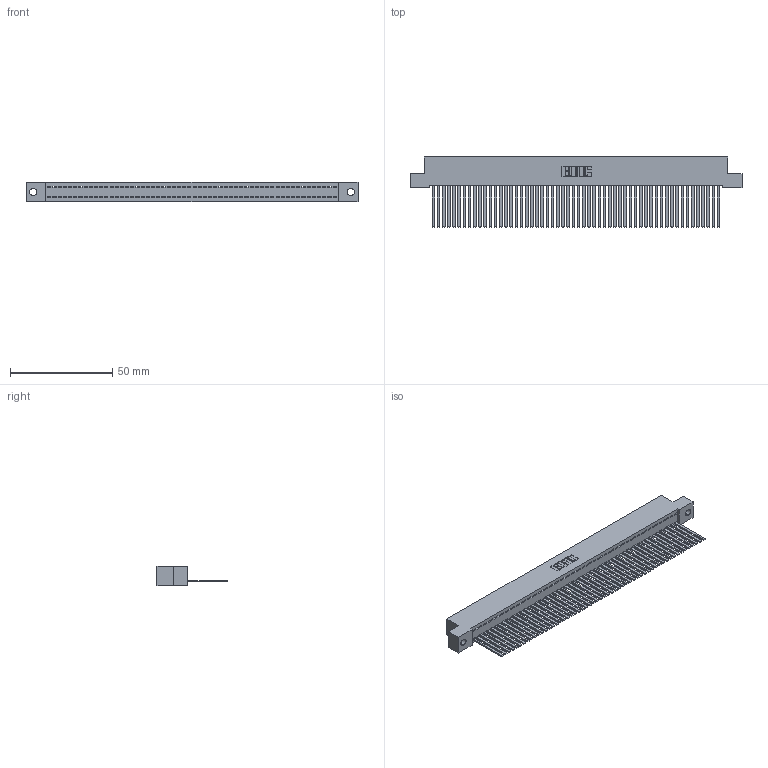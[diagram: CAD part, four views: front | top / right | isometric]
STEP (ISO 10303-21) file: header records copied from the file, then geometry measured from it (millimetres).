
FILE_DESCRIPTION (( 'STEP AP203' ), '1' );
FILE_NAME ('342-056-544-102.STEP', '2019-10-03T11:33:07', ( '' ), ( '' ), 'SwSTEP 2.0', 'SolidWorks 2016', '' );
FILE_SCHEMA (( 'CONFIG_CONTROL_DESIGN' ));
Length unit declared in the file: inch
Products named in the file (3): 345-292-001_345-293-144; 342-056-544-102; 342 Part_.128 Slot
Assembly tree (57 placements, depth 2):
  342-056-544-102
    342 Part_.128 Slot
    345-292-001_345-293-144  x56
Bounding box: 162.56 x 34.3 x 9.4 mm (x, y, z)
Volume: 14901.2 mm3; surface area: 23748.7 mm2
Topology: 57 solids, 57 shells, 3026 faces, 9159 edges, 6030 vertices
Faces by surface type: plane 2198, cylinder 828
Entity records: 32243 total; most frequent: CARTESIAN_POINT 5566, ORIENTED_EDGE 5558, DIRECTION 4663, EDGE_CURVE 2779, VECTOR 2655, LINE 2655, VERTEX_POINT 1850, AXIS2_PLACEMENT_3D 1004
